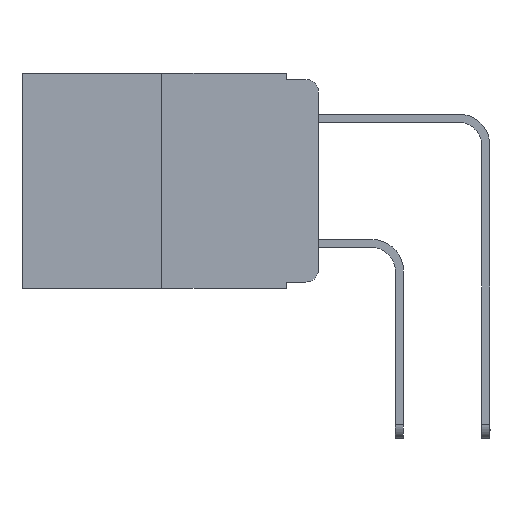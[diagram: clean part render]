
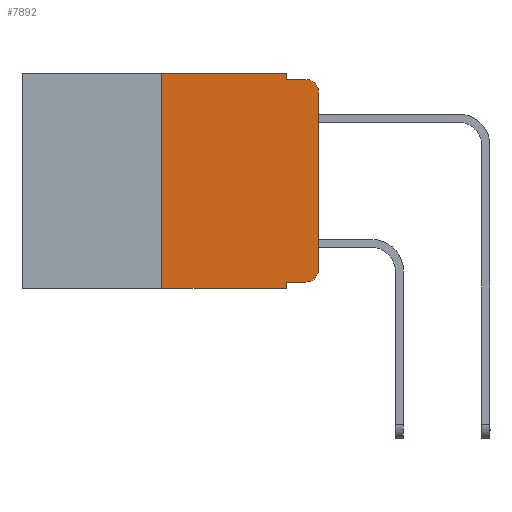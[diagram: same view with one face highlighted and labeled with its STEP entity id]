
A CAD part, left-side view. The second image highlights one B-rep face of the part: STEP entity #7892.
In plain terms, the highlighted planar face has unit normal (-1, 0, 0).
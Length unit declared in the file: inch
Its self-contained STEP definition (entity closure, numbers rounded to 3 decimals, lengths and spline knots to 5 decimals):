
#160 = EDGE_CURVE ( 'NONE', #14895, #15249, #20011, .T. ) ;
#386 = CARTESIAN_POINT ( 'NONE',  ( 0., 0.051, 0. ) ) ;
#470 = VECTOR ( 'NONE', #4839, 39.37008 ) ;
#705 = DIRECTION ( 'NONE',  ( 0., -1., 0. ) ) ;
#758 = VERTEX_POINT ( 'NONE', #24874 ) ;
#1013 = VECTOR ( 'NONE', #10090, 39.37008 ) ;
#1803 = DIRECTION ( 'NONE',  ( 0., -1., 0. ) ) ;
#1981 = EDGE_CURVE ( 'NONE', #22547, #3438, #11292, .T. ) ;
#3057 = CARTESIAN_POINT ( 'NONE',  ( 0., 0., 0. ) ) ;
#3340 = VECTOR ( 'NONE', #5287, 39.37008 ) ;
#3355 = ORIENTED_EDGE ( 'NONE', *, *, #11534, .F. ) ;
#3438 = VERTEX_POINT ( 'NONE', #18893 ) ;
#3591 = ORIENTED_EDGE ( 'NONE', *, *, #160, .F. ) ;
#3881 = ORIENTED_EDGE ( 'NONE', *, *, #21176, .T. ) ;
#4182 = EDGE_CURVE ( 'NONE', #17964, #758, #24291, .T. ) ;
#4184 = DIRECTION ( 'NONE',  ( 0., -1., 0. ) ) ;
#4244 = VERTEX_POINT ( 'NONE', #9369 ) ;
#4839 = DIRECTION ( 'NONE',  ( 0., 0., 1. ) ) ;
#5070 = VERTEX_POINT ( 'NONE', #6743 ) ;
#5287 = DIRECTION ( 'NONE',  ( 0., -1., 0. ) ) ;
#5710 = ORIENTED_EDGE ( 'NONE', *, *, #7002, .T. ) ;
#6075 = DIRECTION ( 'NONE',  ( 0., 0., -1. ) ) ;
#6149 = ORIENTED_EDGE ( 'NONE', *, *, #8722, .T. ) ;
#6261 = EDGE_LOOP ( 'NONE', ( #5710, #11322, #3355, #10349, #16253, #20892, #21533, #3591, #3881, #6149 ) ) ;
#6579 = EDGE_CURVE ( 'NONE', #6682, #5070, #16614, .T. ) ;
#6682 = VERTEX_POINT ( 'NONE', #13681 ) ;
#6743 = CARTESIAN_POINT ( 'NONE',  ( 0., 0.25, 0. ) ) ;
#7002 = EDGE_CURVE ( 'NONE', #4244, #22547, #7834, .T. ) ;
#7126 = DIRECTION ( 'NONE',  ( 0., 0., -1. ) ) ;
#7589 = CARTESIAN_POINT ( 'NONE',  ( 0., 0.051, -0.343 ) ) ;
#7834 = LINE ( 'NONE', #3057, #18929 ) ;
#7892 = ADVANCED_FACE ( 'NONE', ( #24589 ), #18837, .F. ) ;
#8678 = LINE ( 'NONE', #15661, #3340 ) ;
#8722 = EDGE_CURVE ( 'NONE', #18343, #4244, #26121, .T. ) ;
#9369 = CARTESIAN_POINT ( 'NONE',  ( 0., 0., -0.313 ) ) ;
#10090 = DIRECTION ( 'NONE',  ( 0., 0., -1. ) ) ;
#10349 = ORIENTED_EDGE ( 'NONE', *, *, #4182, .F. ) ;
#10941 = DIRECTION ( 'NONE',  ( 1., 0., 0. ) ) ;
#10974 = CARTESIAN_POINT ( 'NONE',  ( 0., 0.051, 0. ) ) ;
#11292 = CIRCLE ( 'NONE', #20550, 0.02 ) ;
#11322 = ORIENTED_EDGE ( 'NONE', *, *, #1981, .T. ) ;
#11534 = EDGE_CURVE ( 'NONE', #758, #3438, #18085, .T. ) ;
#11616 = CARTESIAN_POINT ( 'NONE',  ( 0., 0.02, -0.313 ) ) ;
#11898 = VECTOR ( 'NONE', #7126, 39.37008 ) ;
#12158 = LINE ( 'NONE', #19114, #25185 ) ;
#12378 = EDGE_CURVE ( 'NONE', #6682, #15249, #12158, .T. ) ;
#13681 = CARTESIAN_POINT ( 'NONE',  ( 0., 0.25, -0.343 ) ) ;
#14895 = VERTEX_POINT ( 'NONE', #16952 ) ;
#15249 = VERTEX_POINT ( 'NONE', #7589 ) ;
#15661 = CARTESIAN_POINT ( 'NONE',  ( 0., 0.051, -0.333 ) ) ;
#16253 = ORIENTED_EDGE ( 'NONE', *, *, #22474, .F. ) ;
#16604 = CARTESIAN_POINT ( 'NONE',  ( 0., 0.051, 0. ) ) ;
#16614 = LINE ( 'NONE', #16912, #470 ) ;
#16912 = CARTESIAN_POINT ( 'NONE',  ( 0., 0.25, 0. ) ) ;
#16952 = CARTESIAN_POINT ( 'NONE',  ( 0., 0.051, -0.333 ) ) ;
#17064 = AXIS2_PLACEMENT_3D ( 'NONE', #11616, #19551, #25822 ) ;
#17169 = VECTOR ( 'NONE', #1803, 39.37008 ) ;
#17401 = DIRECTION ( 'NONE',  ( 0., 0., -1. ) ) ;
#17964 = VERTEX_POINT ( 'NONE', #16604 ) ;
#18085 = LINE ( 'NONE', #22564, #19999 ) ;
#18253 = CARTESIAN_POINT ( 'NONE',  ( 0., 0.02, -0.03 ) ) ;
#18343 = VERTEX_POINT ( 'NONE', #23437 ) ;
#18837 = PLANE ( 'NONE',  #20460 ) ;
#18893 = CARTESIAN_POINT ( 'NONE',  ( 0., 0.02, -0.01 ) ) ;
#18929 = VECTOR ( 'NONE', #19260, 39.37008 ) ;
#19114 = CARTESIAN_POINT ( 'NONE',  ( 0., 0.473, -0.343 ) ) ;
#19260 = DIRECTION ( 'NONE',  ( 0., 0., 1. ) ) ;
#19551 = DIRECTION ( 'NONE',  ( -1., 0., 0. ) ) ;
#19940 = CARTESIAN_POINT ( 'NONE',  ( 0., 0., -0.03 ) ) ;
#19999 = VECTOR ( 'NONE', #4184, 39.37008 ) ;
#20011 = LINE ( 'NONE', #386, #1013 ) ;
#20460 = AXIS2_PLACEMENT_3D ( 'NONE', #23090, #10941, #17401 ) ;
#20550 = AXIS2_PLACEMENT_3D ( 'NONE', #18253, #24112, #6075 ) ;
#20892 = ORIENTED_EDGE ( 'NONE', *, *, #6579, .F. ) ;
#21176 = EDGE_CURVE ( 'NONE', #14895, #18343, #8678, .T. ) ;
#21533 = ORIENTED_EDGE ( 'NONE', *, *, #12378, .T. ) ;
#22474 = EDGE_CURVE ( 'NONE', #5070, #17964, #22571, .T. ) ;
#22547 = VERTEX_POINT ( 'NONE', #19940 ) ;
#22564 = CARTESIAN_POINT ( 'NONE',  ( 0., 0.051, -0.01 ) ) ;
#22571 = LINE ( 'NONE', #23841, #17169 ) ;
#23090 = CARTESIAN_POINT ( 'NONE',  ( 0., 0.473, 0. ) ) ;
#23437 = CARTESIAN_POINT ( 'NONE',  ( 0., 0.02, -0.333 ) ) ;
#23841 = CARTESIAN_POINT ( 'NONE',  ( 0., 0.473, 0. ) ) ;
#24112 = DIRECTION ( 'NONE',  ( -1., 0., 0. ) ) ;
#24291 = LINE ( 'NONE', #10974, #11898 ) ;
#24589 = FACE_OUTER_BOUND ( 'NONE', #6261, .T. ) ;
#24874 = CARTESIAN_POINT ( 'NONE',  ( 0., 0.051, -0.01 ) ) ;
#25185 = VECTOR ( 'NONE', #705, 39.37008 ) ;
#25822 = DIRECTION ( 'NONE',  ( 0., 0., -1. ) ) ;
#26121 = CIRCLE ( 'NONE', #17064, 0.02 ) ;
